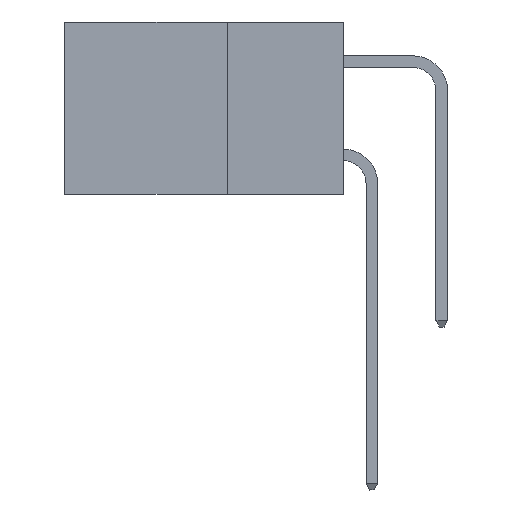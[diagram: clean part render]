
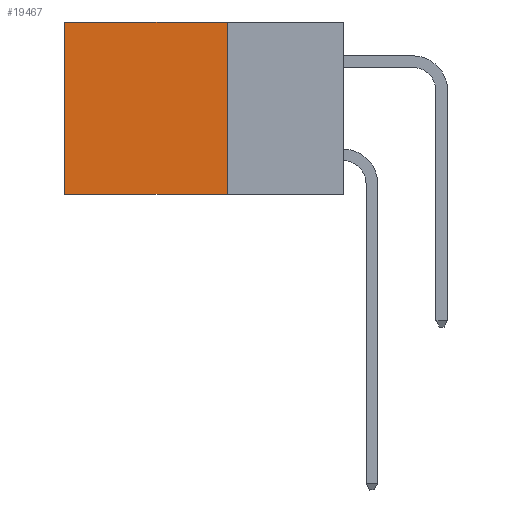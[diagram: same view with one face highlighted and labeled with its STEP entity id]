
A CAD part, left-side view. The second image highlights one B-rep face of the part: STEP entity #19467.
In plain terms, the highlighted planar face has unit normal (-1, 0, 0).
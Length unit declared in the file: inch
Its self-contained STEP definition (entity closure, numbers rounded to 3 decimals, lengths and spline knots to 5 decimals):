
#126 = DIRECTION ( 'NONE',  ( 1., 0., 0. ) ) ;
#354 = VECTOR ( 'NONE', #15244, 39.37008 ) ;
#2074 = DIRECTION ( 'NONE',  ( 0., 1., 0. ) ) ;
#2306 = VECTOR ( 'NONE', #8883, 39.37008 ) ;
#3565 = VERTEX_POINT ( 'NONE', #8865 ) ;
#4164 = CARTESIAN_POINT ( 'NONE',  ( 0.2615, 0.6, -0.37 ) ) ;
#5371 = VERTEX_POINT ( 'NONE', #8622 ) ;
#6969 = EDGE_CURVE ( 'NONE', #3565, #8966, #12870, .T. ) ;
#7202 = ORIENTED_EDGE ( 'NONE', *, *, #9958, .T. ) ;
#7604 = EDGE_CURVE ( 'NONE', #21815, #5371, #15446, .T. ) ;
#7838 = CARTESIAN_POINT ( 'NONE',  ( 0.2615, 0.25, -0.37 ) ) ;
#8355 = VECTOR ( 'NONE', #2074, 39.37008 ) ;
#8622 = CARTESIAN_POINT ( 'NONE',  ( 0.2615, 0.6, -0.37 ) ) ;
#8638 = CARTESIAN_POINT ( 'NONE',  ( 0.2615, 0.25, 0. ) ) ;
#8865 = CARTESIAN_POINT ( 'NONE',  ( 0.2615, 0.25, 0. ) ) ;
#8883 = DIRECTION ( 'NONE',  ( 0., 0., -1. ) ) ;
#8936 = LINE ( 'NONE', #7838, #8355 ) ;
#8966 = VERTEX_POINT ( 'NONE', #11620 ) ;
#9438 = FACE_OUTER_BOUND ( 'NONE', #23237, .T. ) ;
#9958 = EDGE_CURVE ( 'NONE', #3565, #21815, #19016, .T. ) ;
#11209 = EDGE_CURVE ( 'NONE', #8966, #5371, #8936, .T. ) ;
#11620 = CARTESIAN_POINT ( 'NONE',  ( 0.2615, 0.25, -0.37 ) ) ;
#12475 = CARTESIAN_POINT ( 'NONE',  ( 0.2615, 0.25, -0.37 ) ) ;
#12787 = ORIENTED_EDGE ( 'NONE', *, *, #11209, .F. ) ;
#12870 = LINE ( 'NONE', #12475, #2306 ) ;
#13418 = DIRECTION ( 'NONE',  ( 0., 0., -1. ) ) ;
#15244 = DIRECTION ( 'NONE',  ( 0., 0., -1. ) ) ;
#15446 = LINE ( 'NONE', #4164, #354 ) ;
#16631 = AXIS2_PLACEMENT_3D ( 'NONE', #22544, #126, #13418 ) ;
#17160 = ORIENTED_EDGE ( 'NONE', *, *, #6969, .F. ) ;
#19016 = LINE ( 'NONE', #8638, #23891 ) ;
#19467 = ADVANCED_FACE ( 'NONE', ( #9438 ), #20703, .F. ) ;
#19824 = CARTESIAN_POINT ( 'NONE',  ( 0.2615, 0.6, 0. ) ) ;
#20703 = PLANE ( 'NONE',  #16631 ) ;
#21467 = DIRECTION ( 'NONE',  ( 0., 1., 0. ) ) ;
#21815 = VERTEX_POINT ( 'NONE', #19824 ) ;
#21966 = ORIENTED_EDGE ( 'NONE', *, *, #7604, .T. ) ;
#22544 = CARTESIAN_POINT ( 'NONE',  ( 0.2615, 0.25, -0.37 ) ) ;
#23237 = EDGE_LOOP ( 'NONE', ( #21966, #12787, #17160, #7202 ) ) ;
#23891 = VECTOR ( 'NONE', #21467, 39.37008 ) ;
